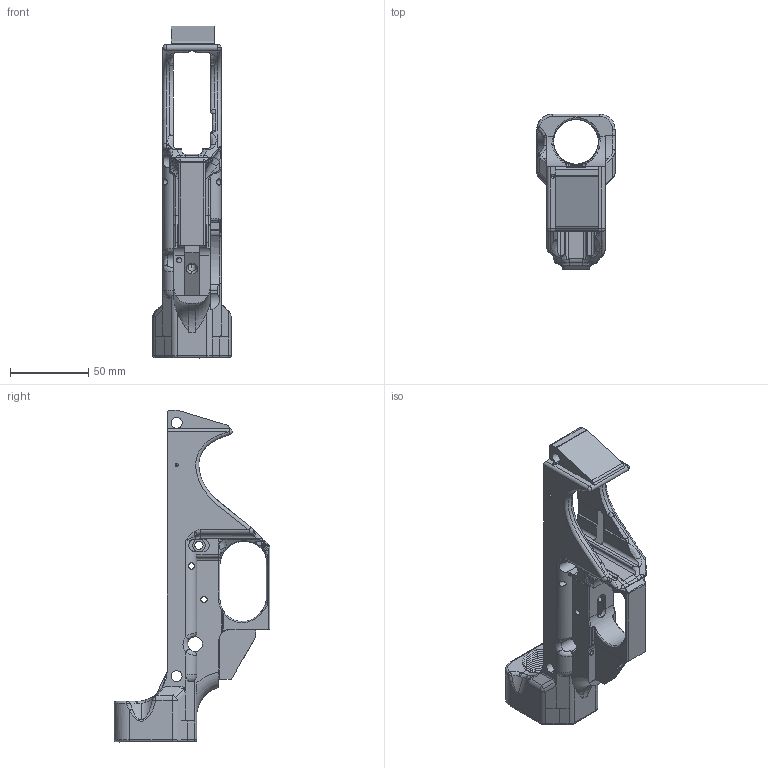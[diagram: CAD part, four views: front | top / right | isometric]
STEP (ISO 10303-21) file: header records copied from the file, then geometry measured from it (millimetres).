
FILE_DESCRIPTION (( 'STEP AP214' ), '1' );
FILE_NAME ('Hermes_v1.4.STEP', '2015-05-21T07:11:22', ( 'WarFairy' ), ( '' ), 'SwSTEP 2.0', 'SolidWorks 2015', '' );
FILE_SCHEMA (( 'AUTOMOTIVE_DESIGN' ));
Length unit declared in the file: inch
Products named in the file (1): Hermes_v1.4
Bounding box: 50 x 99.72 x 212.24 mm (x, y, z)
Volume: 166804.5 mm3; surface area: 55939.7 mm2
Topology: 1 solids, 3 shells, 597 faces, 1681 edges, 1054 vertices
Faces by surface type: cylinder 243, bspline 174, plane 124, torus 38, sphere 9, cone 9
Entity records: 45093 total; most frequent: CARTESIAN_POINT 31591, ORIENTED_EDGE 3308, DIRECTION 2190, EDGE_CURVE 1654, VERTEX_POINT 1054, AXIS2_PLACEMENT_3D 837, B_SPLINE_CURVE_WITH_KNOTS 644, EDGE_LOOP 626
